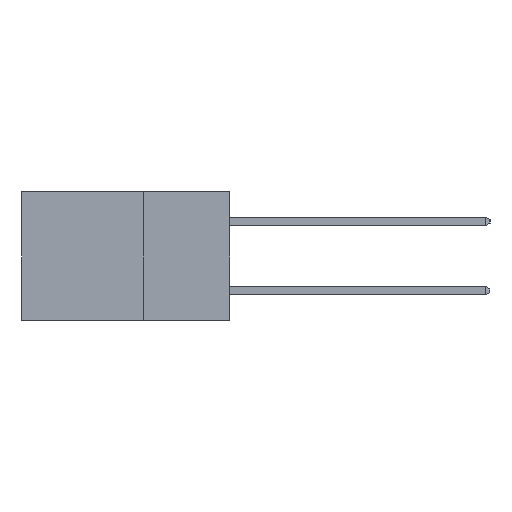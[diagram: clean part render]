
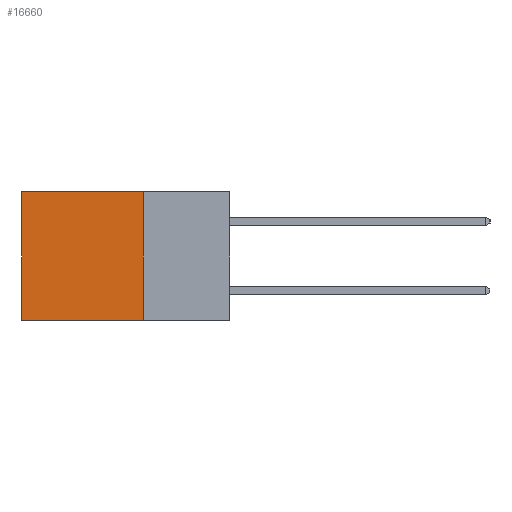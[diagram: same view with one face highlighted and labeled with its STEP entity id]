
A CAD part, left-side view. The second image highlights one B-rep face of the part: STEP entity #16660.
In plain terms, the highlighted planar face has unit normal (-1, 0, 0).
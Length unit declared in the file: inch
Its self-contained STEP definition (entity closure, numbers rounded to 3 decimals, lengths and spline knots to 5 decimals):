
#387 = EDGE_CURVE ( 'NONE', #8617, #21715, #5764, .T. ) ;
#3506 = CARTESIAN_POINT ( 'NONE',  ( 0.2615, 0.25, -0.37 ) ) ;
#4054 = CARTESIAN_POINT ( 'NONE',  ( 0.2615, 0.25, -0.37 ) ) ;
#4225 = VECTOR ( 'NONE', #6477, 39.37008 ) ;
#4425 = VECTOR ( 'NONE', #20574, 39.37008 ) ;
#5094 = LINE ( 'NONE', #10401, #26208 ) ;
#5610 = DIRECTION ( 'NONE',  ( 1., 0., 0. ) ) ;
#5764 = LINE ( 'NONE', #14072, #4425 ) ;
#6477 = DIRECTION ( 'NONE',  ( 0., 0., -1. ) ) ;
#6693 = CARTESIAN_POINT ( 'NONE',  ( 0.2615, 0.25, -0.37 ) ) ;
#7546 = VECTOR ( 'NONE', #18459, 39.37008 ) ;
#8617 = VERTEX_POINT ( 'NONE', #6693 ) ;
#10401 = CARTESIAN_POINT ( 'NONE',  ( 0.2615, 0.25, 0. ) ) ;
#11872 = CARTESIAN_POINT ( 'NONE',  ( 0.2615, 0.6, -0.37 ) ) ;
#13028 = LINE ( 'NONE', #4054, #7546 ) ;
#13091 = ORIENTED_EDGE ( 'NONE', *, *, #15283, .T. ) ;
#14023 = FACE_OUTER_BOUND ( 'NONE', #23940, .T. ) ;
#14072 = CARTESIAN_POINT ( 'NONE',  ( 0.2615, 0.25, -0.37 ) ) ;
#14670 = CARTESIAN_POINT ( 'NONE',  ( 0.2615, 0.6, -0.37 ) ) ;
#14968 = CARTESIAN_POINT ( 'NONE',  ( 0.2615, 0.6, 0. ) ) ;
#15283 = EDGE_CURVE ( 'NONE', #26019, #21715, #21252, .T. ) ;
#15883 = PLANE ( 'NONE',  #24985 ) ;
#16124 = ORIENTED_EDGE ( 'NONE', *, *, #22503, .F. ) ;
#16660 = ADVANCED_FACE ( 'NONE', ( #14023 ), #15883, .F. ) ;
#17626 = CARTESIAN_POINT ( 'NONE',  ( 0.2615, 0.25, 0. ) ) ;
#18459 = DIRECTION ( 'NONE',  ( 0., 0., -1. ) ) ;
#18632 = VERTEX_POINT ( 'NONE', #17626 ) ;
#19217 = ORIENTED_EDGE ( 'NONE', *, *, #387, .F. ) ;
#19932 = DIRECTION ( 'NONE',  ( 0., 0., -1. ) ) ;
#20535 = ORIENTED_EDGE ( 'NONE', *, *, #20555, .T. ) ;
#20555 = EDGE_CURVE ( 'NONE', #18632, #26019, #5094, .T. ) ;
#20574 = DIRECTION ( 'NONE',  ( 0., 1., 0. ) ) ;
#20665 = DIRECTION ( 'NONE',  ( 0., 1., 0. ) ) ;
#21252 = LINE ( 'NONE', #14670, #4225 ) ;
#21715 = VERTEX_POINT ( 'NONE', #11872 ) ;
#22503 = EDGE_CURVE ( 'NONE', #18632, #8617, #13028, .T. ) ;
#23940 = EDGE_LOOP ( 'NONE', ( #13091, #19217, #16124, #20535 ) ) ;
#24985 = AXIS2_PLACEMENT_3D ( 'NONE', #3506, #5610, #19932 ) ;
#26019 = VERTEX_POINT ( 'NONE', #14968 ) ;
#26208 = VECTOR ( 'NONE', #20665, 39.37008 ) ;
